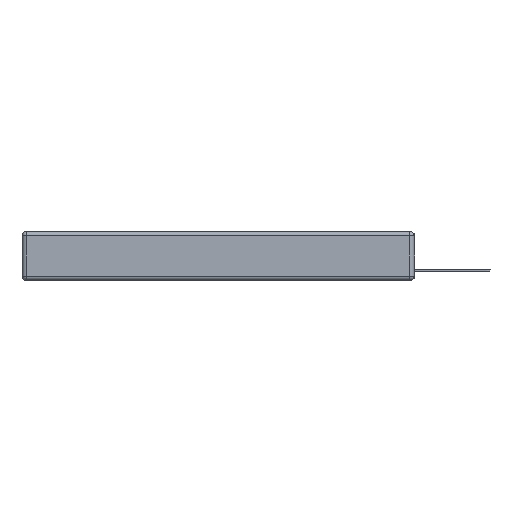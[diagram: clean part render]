
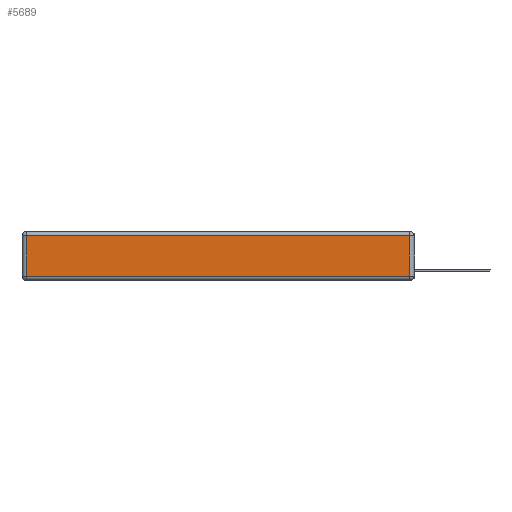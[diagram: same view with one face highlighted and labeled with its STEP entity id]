
A CAD part, left-side view. The second image highlights one B-rep face of the part: STEP entity #5689.
In plain terms, the highlighted planar face has unit normal (-1, 0, 0).
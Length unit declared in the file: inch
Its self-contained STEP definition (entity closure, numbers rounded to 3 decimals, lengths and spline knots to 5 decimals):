
#1448 = VERTEX_POINT ( 'NONE', #11196 ) ;
#1521 = VECTOR ( 'NONE', #16549, 39.37008 ) ;
#2274 = CARTESIAN_POINT ( 'NONE',  ( 0., 2.72, -0.03 ) ) ;
#2552 = DIRECTION ( 'NONE',  ( 0., 0., 1. ) ) ;
#3101 = LINE ( 'NONE', #12738, #1521 ) ;
#3233 = DIRECTION ( 'NONE',  ( 0., 0., -1. ) ) ;
#3271 = EDGE_LOOP ( 'NONE', ( #15780, #9866, #6102, #16416 ) ) ;
#4124 = EDGE_CURVE ( 'NONE', #11848, #14418, #3101, .T. ) ;
#4433 = EDGE_CURVE ( 'NONE', #1448, #15401, #5633, .T. ) ;
#4814 = EDGE_CURVE ( 'NONE', #14418, #1448, #10881, .T. ) ;
#5589 = VECTOR ( 'NONE', #2552, 39.37008 ) ;
#5633 = LINE ( 'NONE', #7123, #13157 ) ;
#5635 = PLANE ( 'NONE',  #7766 ) ;
#5689 = ADVANCED_FACE ( 'NONE', ( #12062 ), #5635, .T. ) ;
#6102 = ORIENTED_EDGE ( 'NONE', *, *, #4433, .T. ) ;
#6732 = DIRECTION ( 'NONE',  ( 0., 0., 1. ) ) ;
#7041 = LINE ( 'NONE', #13494, #10595 ) ;
#7123 = CARTESIAN_POINT ( 'NONE',  ( 0., 2.75, -0.03 ) ) ;
#7138 = CARTESIAN_POINT ( 'NONE',  ( 0., 2.72, -0.313 ) ) ;
#7766 = AXIS2_PLACEMENT_3D ( 'NONE', #10771, #15960, #6732 ) ;
#9866 = ORIENTED_EDGE ( 'NONE', *, *, #4814, .T. ) ;
#10595 = VECTOR ( 'NONE', #3233, 39.37008 ) ;
#10771 = CARTESIAN_POINT ( 'NONE',  ( 0., 0., -0.343 ) ) ;
#10881 = LINE ( 'NONE', #16073, #5589 ) ;
#11196 = CARTESIAN_POINT ( 'NONE',  ( 0., 0.03, -0.03 ) ) ;
#11848 = VERTEX_POINT ( 'NONE', #7138 ) ;
#12062 = FACE_OUTER_BOUND ( 'NONE', #3271, .T. ) ;
#12161 = EDGE_CURVE ( 'NONE', #15401, #11848, #7041, .T. ) ;
#12738 = CARTESIAN_POINT ( 'NONE',  ( 0., 0., -0.313 ) ) ;
#13157 = VECTOR ( 'NONE', #14683, 39.37008 ) ;
#13296 = CARTESIAN_POINT ( 'NONE',  ( 0., 0.03, -0.313 ) ) ;
#13494 = CARTESIAN_POINT ( 'NONE',  ( 0., 2.72, -0.343 ) ) ;
#14418 = VERTEX_POINT ( 'NONE', #13296 ) ;
#14683 = DIRECTION ( 'NONE',  ( 0., 1., 0. ) ) ;
#15401 = VERTEX_POINT ( 'NONE', #2274 ) ;
#15780 = ORIENTED_EDGE ( 'NONE', *, *, #4124, .T. ) ;
#15960 = DIRECTION ( 'NONE',  ( -1., 0., 0. ) ) ;
#16073 = CARTESIAN_POINT ( 'NONE',  ( 0., 0.03, -0.343 ) ) ;
#16416 = ORIENTED_EDGE ( 'NONE', *, *, #12161, .T. ) ;
#16549 = DIRECTION ( 'NONE',  ( 0., -1., 0. ) ) ;
